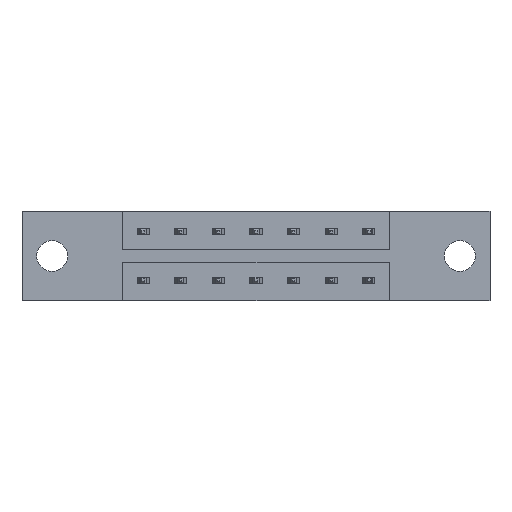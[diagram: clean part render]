
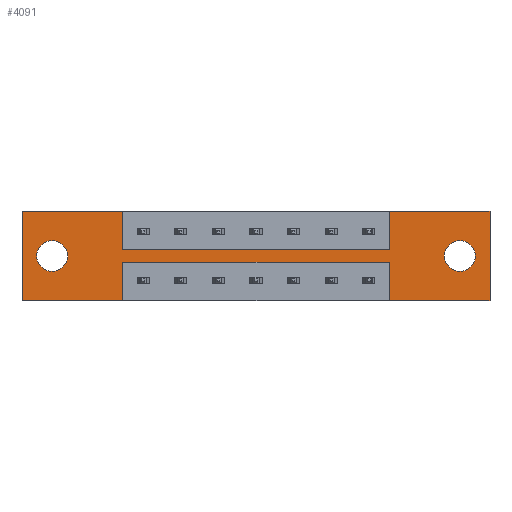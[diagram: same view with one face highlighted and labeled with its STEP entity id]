
A CAD part, front view. The second image highlights one B-rep face of the part: STEP entity #4091.
In plain terms, the highlighted planar face has unit normal (0, -1, 0).
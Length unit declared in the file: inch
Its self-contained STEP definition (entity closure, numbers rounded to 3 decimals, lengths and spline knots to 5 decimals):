
#109 = DIRECTION ( 'NONE',  ( 1., 0., 0. ) ) ;
#165 = DIRECTION ( 'NONE',  ( -1., 0., 0. ) ) ;
#204 = DIRECTION ( 'NONE',  ( 0., 0., 1. ) ) ;
#214 = VERTEX_POINT ( 'NONE', #8404 ) ;
#340 = EDGE_CURVE ( 'NONE', #2981, #5313, #6442, .T. ) ;
#433 = VECTOR ( 'NONE', #8937, 39.37008 ) ;
#441 = EDGE_CURVE ( 'NONE', #3346, #5144, #3145, .T. ) ;
#467 = EDGE_CURVE ( 'NONE', #1320, #6715, #2736, .T. ) ;
#503 = EDGE_CURVE ( 'NONE', #4064, #1999, #2472, .T. ) ;
#505 = EDGE_CURVE ( 'NONE', #4985, #8348, #5949, .T. ) ;
#507 = LINE ( 'NONE', #5925, #7825 ) ;
#518 = EDGE_CURVE ( 'NONE', #5144, #4828, #3897, .T. ) ;
#522 = EDGE_CURVE ( 'NONE', #7016, #8279, #2224, .T. ) ;
#539 = EDGE_CURVE ( 'NONE', #6483, #7016, #4149, .T. ) ;
#541 = EDGE_CURVE ( 'NONE', #5313, #6483, #5565, .T. ) ;
#542 = EDGE_CURVE ( 'NONE', #214, #1320, #8900, .T. ) ;
#552 = EDGE_CURVE ( 'NONE', #4828, #214, #6865, .T. ) ;
#567 = VECTOR ( 'NONE', #6839, 39.37008 ) ;
#651 = VECTOR ( 'NONE', #3883, 39.37008 ) ;
#670 = PLANE ( 'NONE',  #3630 ) ;
#857 = ORIENTED_EDGE ( 'NONE', *, *, #6706, .F. ) ;
#930 = LINE ( 'NONE', #6050, #651 ) ;
#1096 = LINE ( 'NONE', #8623, #4838 ) ;
#1152 = ORIENTED_EDGE ( 'NONE', *, *, #340, .F. ) ;
#1211 = CARTESIAN_POINT ( 'NONE',  ( 1.5225, 0., -0.1585 ) ) ;
#1237 = CARTESIAN_POINT ( 'NONE',  ( 1.94, 0., 0. ) ) ;
#1270 = EDGE_CURVE ( 'NONE', #1999, #4064, #5923, .T. ) ;
#1320 = VERTEX_POINT ( 'NONE', #2807 ) ;
#1342 = FACE_BOUND ( 'NONE', #8694, .T. ) ;
#1357 = EDGE_CURVE ( 'NONE', #8348, #4985, #8129, .T. ) ;
#1390 = ORIENTED_EDGE ( 'NONE', *, *, #552, .F. ) ;
#1520 = DIRECTION ( 'NONE',  ( 0., 0., -1. ) ) ;
#1537 = DIRECTION ( 'NONE',  ( 0., 1., 0. ) ) ;
#1668 = CARTESIAN_POINT ( 'NONE',  ( 0.125, 0., -0.185 ) ) ;
#1776 = EDGE_CURVE ( 'NONE', #8279, #7370, #930, .T. ) ;
#1842 = CARTESIAN_POINT ( 'NONE',  ( 1.5225, 0., 0. ) ) ;
#1999 = VERTEX_POINT ( 'NONE', #8485 ) ;
#2007 = VECTOR ( 'NONE', #6597, 39.37008 ) ;
#2095 = CARTESIAN_POINT ( 'NONE',  ( 1.815, 0., -0.185 ) ) ;
#2224 = LINE ( 'NONE', #1211, #5747 ) ;
#2460 = DIRECTION ( 'NONE',  ( 0., 0., -1. ) ) ;
#2472 = CIRCLE ( 'NONE', #8506, 0.064 ) ;
#2505 = CARTESIAN_POINT ( 'NONE',  ( 0.4175, 0., 0. ) ) ;
#2563 = DIRECTION ( 'NONE',  ( -1., 0., 0. ) ) ;
#2736 = LINE ( 'NONE', #4361, #567 ) ;
#2807 = CARTESIAN_POINT ( 'NONE',  ( 0.4175, 0., -0.37 ) ) ;
#2875 = DIRECTION ( 'NONE',  ( 0., 0., 1. ) ) ;
#2957 = ORIENTED_EDGE ( 'NONE', *, *, #1776, .F. ) ;
#2981 = VERTEX_POINT ( 'NONE', #5919 ) ;
#3085 = AXIS2_PLACEMENT_3D ( 'NONE', #1668, #1537, #2875 ) ;
#3145 = LINE ( 'NONE', #6995, #6541 ) ;
#3150 = ORIENTED_EDGE ( 'NONE', *, *, #5723, .F. ) ;
#3177 = CARTESIAN_POINT ( 'NONE',  ( 0., 0., -0.37 ) ) ;
#3346 = VERTEX_POINT ( 'NONE', #4205 ) ;
#3611 = AXIS2_PLACEMENT_3D ( 'NONE', #6206, #8874, #8891 ) ;
#3630 = AXIS2_PLACEMENT_3D ( 'NONE', #8928, #3671, #1520 ) ;
#3653 = VECTOR ( 'NONE', #109, 39.37008 ) ;
#3671 = DIRECTION ( 'NONE',  ( 0., -1., 0. ) ) ;
#3883 = DIRECTION ( 'NONE',  ( 1., 0., 0. ) ) ;
#3897 = LINE ( 'NONE', #4693, #2007 ) ;
#4033 = CARTESIAN_POINT ( 'NONE',  ( 0.125, 0., -0.249 ) ) ;
#4064 = VERTEX_POINT ( 'NONE', #6338 ) ;
#4091 = ADVANCED_FACE ( 'NONE', ( #1342, #6508, #6945 ), #670, .T. ) ;
#4149 = LINE ( 'NONE', #8909, #3653 ) ;
#4205 = CARTESIAN_POINT ( 'NONE',  ( 1.94, 0., -0.37 ) ) ;
#4361 = CARTESIAN_POINT ( 'NONE',  ( 0., 0., -0.37 ) ) ;
#4392 = ORIENTED_EDGE ( 'NONE', *, *, #503, .T. ) ;
#4599 = CARTESIAN_POINT ( 'NONE',  ( 0.125, 0., -0.121 ) ) ;
#4648 = ORIENTED_EDGE ( 'NONE', *, *, #1357, .T. ) ;
#4693 = CARTESIAN_POINT ( 'NONE',  ( 1.5225, 0., -0.2115 ) ) ;
#4728 = DIRECTION ( 'NONE',  ( 0., 0., -1. ) ) ;
#4828 = VERTEX_POINT ( 'NONE', #5851 ) ;
#4838 = VECTOR ( 'NONE', #204, 39.37008 ) ;
#4881 = ORIENTED_EDGE ( 'NONE', *, *, #522, .F. ) ;
#4985 = VERTEX_POINT ( 'NONE', #4599 ) ;
#5072 = ORIENTED_EDGE ( 'NONE', *, *, #467, .F. ) ;
#5144 = VERTEX_POINT ( 'NONE', #8458 ) ;
#5156 = VECTOR ( 'NONE', #165, 39.37008 ) ;
#5313 = VERTEX_POINT ( 'NONE', #2505 ) ;
#5354 = VECTOR ( 'NONE', #4728, 39.37008 ) ;
#5565 = LINE ( 'NONE', #8296, #8729 ) ;
#5723 = EDGE_CURVE ( 'NONE', #6715, #2981, #1096, .T. ) ;
#5747 = VECTOR ( 'NONE', #8309, 39.37008 ) ;
#5851 = CARTESIAN_POINT ( 'NONE',  ( 1.5225, 0., -0.2115 ) ) ;
#5919 = CARTESIAN_POINT ( 'NONE',  ( 0., 0., 0. ) ) ;
#5923 = CIRCLE ( 'NONE', #3611, 0.064 ) ;
#5925 = CARTESIAN_POINT ( 'NONE',  ( 1.94, 0., 0. ) ) ;
#5949 = CIRCLE ( 'NONE', #8490, 0.064 ) ;
#6050 = CARTESIAN_POINT ( 'NONE',  ( 0., 0., 0. ) ) ;
#6156 = ORIENTED_EDGE ( 'NONE', *, *, #1270, .T. ) ;
#6206 = CARTESIAN_POINT ( 'NONE',  ( 1.815, 0., -0.185 ) ) ;
#6338 = CARTESIAN_POINT ( 'NONE',  ( 1.815, 0., -0.121 ) ) ;
#6343 = ORIENTED_EDGE ( 'NONE', *, *, #518, .F. ) ;
#6442 = LINE ( 'NONE', #7083, #433 ) ;
#6483 = VERTEX_POINT ( 'NONE', #8342 ) ;
#6508 = FACE_BOUND ( 'NONE', #7103, .T. ) ;
#6541 = VECTOR ( 'NONE', #2563, 39.37008 ) ;
#6547 = ORIENTED_EDGE ( 'NONE', *, *, #539, .F. ) ;
#6597 = DIRECTION ( 'NONE',  ( 0., 0., 1. ) ) ;
#6631 = DIRECTION ( 'NONE',  ( 0., 0., -1. ) ) ;
#6706 = EDGE_CURVE ( 'NONE', #7370, #3346, #507, .T. ) ;
#6715 = VERTEX_POINT ( 'NONE', #3177 ) ;
#6778 = DIRECTION ( 'NONE',  ( 0., 0., 1. ) ) ;
#6839 = DIRECTION ( 'NONE',  ( -1., 0., 0. ) ) ;
#6865 = LINE ( 'NONE', #7585, #5156 ) ;
#6945 = FACE_OUTER_BOUND ( 'NONE', #7114, .T. ) ;
#6952 = DIRECTION ( 'NONE',  ( 0., 1., 0. ) ) ;
#6995 = CARTESIAN_POINT ( 'NONE',  ( 0., 0., -0.37 ) ) ;
#7004 = CARTESIAN_POINT ( 'NONE',  ( 0.125, 0., -0.185 ) ) ;
#7016 = VERTEX_POINT ( 'NONE', #8612 ) ;
#7083 = CARTESIAN_POINT ( 'NONE',  ( 0., 0., 0. ) ) ;
#7103 = EDGE_LOOP ( 'NONE', ( #7880, #4648 ) ) ;
#7114 = EDGE_LOOP ( 'NONE', ( #6343, #8071, #857, #2957, #4881, #6547, #8246, #1152, #3150, #5072, #8434, #1390 ) ) ;
#7370 = VERTEX_POINT ( 'NONE', #1237 ) ;
#7457 = DIRECTION ( 'NONE',  ( 0., 1., 0. ) ) ;
#7585 = CARTESIAN_POINT ( 'NONE',  ( 0.4175, 0., -0.2115 ) ) ;
#7825 = VECTOR ( 'NONE', #2460, 39.37008 ) ;
#7880 = ORIENTED_EDGE ( 'NONE', *, *, #505, .T. ) ;
#8071 = ORIENTED_EDGE ( 'NONE', *, *, #441, .F. ) ;
#8129 = CIRCLE ( 'NONE', #3085, 0.064 ) ;
#8246 = ORIENTED_EDGE ( 'NONE', *, *, #541, .F. ) ;
#8279 = VERTEX_POINT ( 'NONE', #1842 ) ;
#8296 = CARTESIAN_POINT ( 'NONE',  ( 0.4175, 0., -0.1585 ) ) ;
#8309 = DIRECTION ( 'NONE',  ( 0., 0., 1. ) ) ;
#8342 = CARTESIAN_POINT ( 'NONE',  ( 0.4175, 0., -0.1585 ) ) ;
#8348 = VERTEX_POINT ( 'NONE', #4033 ) ;
#8404 = CARTESIAN_POINT ( 'NONE',  ( 0.4175, 0., -0.2115 ) ) ;
#8434 = ORIENTED_EDGE ( 'NONE', *, *, #542, .F. ) ;
#8458 = CARTESIAN_POINT ( 'NONE',  ( 1.5225, 0., -0.37 ) ) ;
#8485 = CARTESIAN_POINT ( 'NONE',  ( 1.815, 0., -0.249 ) ) ;
#8490 = AXIS2_PLACEMENT_3D ( 'NONE', #7004, #6952, #6778 ) ;
#8506 = AXIS2_PLACEMENT_3D ( 'NONE', #2095, #7457, #6631 ) ;
#8612 = CARTESIAN_POINT ( 'NONE',  ( 1.5225, 0., -0.1585 ) ) ;
#8623 = CARTESIAN_POINT ( 'NONE',  ( 0., 0., 0. ) ) ;
#8694 = EDGE_LOOP ( 'NONE', ( #4392, #6156 ) ) ;
#8729 = VECTOR ( 'NONE', #9044, 39.37008 ) ;
#8804 = CARTESIAN_POINT ( 'NONE',  ( 0.4175, 0., -0.2115 ) ) ;
#8874 = DIRECTION ( 'NONE',  ( 0., 1., 0. ) ) ;
#8891 = DIRECTION ( 'NONE',  ( 0., 0., -1. ) ) ;
#8900 = LINE ( 'NONE', #8804, #5354 ) ;
#8909 = CARTESIAN_POINT ( 'NONE',  ( 0.4175, 0., -0.1585 ) ) ;
#8928 = CARTESIAN_POINT ( 'NONE',  ( 0., 0., -0.37 ) ) ;
#8937 = DIRECTION ( 'NONE',  ( 1., 0., 0. ) ) ;
#9044 = DIRECTION ( 'NONE',  ( 0., 0., -1. ) ) ;
